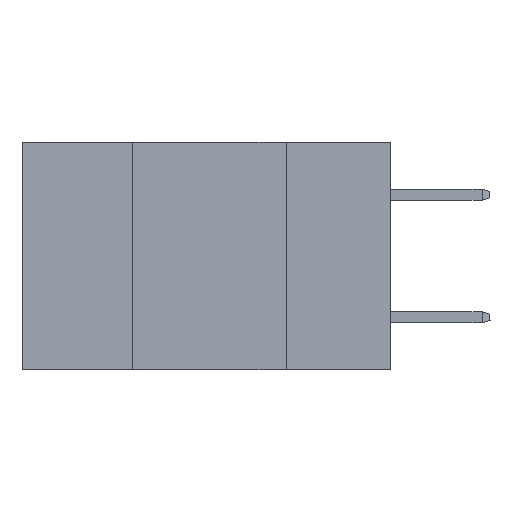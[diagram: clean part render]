
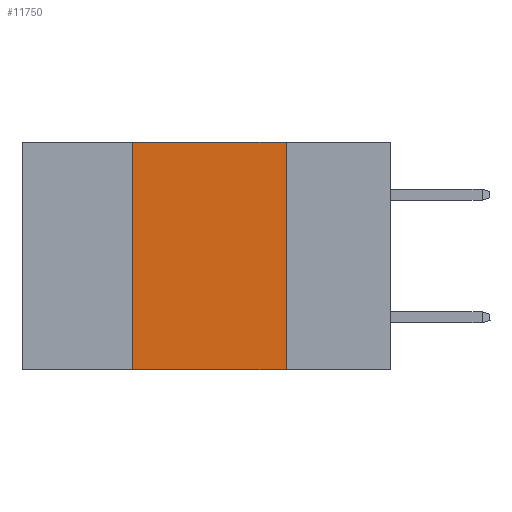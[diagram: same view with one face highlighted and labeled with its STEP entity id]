
A CAD part, left-side view. The second image highlights one B-rep face of the part: STEP entity #11750.
In plain terms, the highlighted planar face has unit normal (-1, 0, 0).
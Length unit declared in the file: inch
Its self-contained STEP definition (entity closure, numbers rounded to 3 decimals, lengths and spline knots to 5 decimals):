
#91 = VERTEX_POINT ( 'NONE', #8208 ) ;
#491 = VECTOR ( 'NONE', #9722, 39.37008 ) ;
#509 = DIRECTION ( 'NONE',  ( 0., -1., 0. ) ) ;
#1171 = LINE ( 'NONE', #6348, #491 ) ;
#2703 = CARTESIAN_POINT ( 'NONE',  ( 0., 0.6, 0. ) ) ;
#2993 = VECTOR ( 'NONE', #509, 39.37008 ) ;
#3059 = DIRECTION ( 'NONE',  ( 0., 0., 1. ) ) ;
#3501 = AXIS2_PLACEMENT_3D ( 'NONE', #6373, #5384, #10749 ) ;
#3661 = VERTEX_POINT ( 'NONE', #12214 ) ;
#5212 = VERTEX_POINT ( 'NONE', #7196 ) ;
#5314 = EDGE_CURVE ( 'NONE', #91, #3661, #13620, .T. ) ;
#5384 = DIRECTION ( 'NONE',  ( 1., 0., 0. ) ) ;
#5668 = PLANE ( 'NONE',  #3501 ) ;
#6065 = EDGE_CURVE ( 'NONE', #3661, #7696, #1171, .T. ) ;
#6348 = CARTESIAN_POINT ( 'NONE',  ( 0., 0.17, 0. ) ) ;
#6373 = CARTESIAN_POINT ( 'NONE',  ( 0., 0.6, 0. ) ) ;
#6686 = ORIENTED_EDGE ( 'NONE', *, *, #10140, .T. ) ;
#7186 = CARTESIAN_POINT ( 'NONE',  ( 0., 0.17, -0.37 ) ) ;
#7196 = CARTESIAN_POINT ( 'NONE',  ( 0., 0.42, -0.37 ) ) ;
#7440 = LINE ( 'NONE', #13830, #12076 ) ;
#7696 = VERTEX_POINT ( 'NONE', #7186 ) ;
#7822 = ORIENTED_EDGE ( 'NONE', *, *, #8713, .F. ) ;
#7993 = VECTOR ( 'NONE', #13829, 39.37008 ) ;
#8208 = CARTESIAN_POINT ( 'NONE',  ( 0., 0.42, 0. ) ) ;
#8713 = EDGE_CURVE ( 'NONE', #5212, #91, #7440, .T. ) ;
#9385 = CARTESIAN_POINT ( 'NONE',  ( 0., 0.6, -0.37 ) ) ;
#9722 = DIRECTION ( 'NONE',  ( 0., 0., -1. ) ) ;
#10140 = EDGE_CURVE ( 'NONE', #5212, #7696, #11594, .T. ) ;
#10749 = DIRECTION ( 'NONE',  ( 0., 0., -1. ) ) ;
#11594 = LINE ( 'NONE', #9385, #7993 ) ;
#11750 = ADVANCED_FACE ( 'NONE', ( #11816 ), #5668, .F. ) ;
#11816 = FACE_OUTER_BOUND ( 'NONE', #13566, .T. ) ;
#12076 = VECTOR ( 'NONE', #3059, 39.37008 ) ;
#12214 = CARTESIAN_POINT ( 'NONE',  ( 0., 0.17, 0. ) ) ;
#12694 = ORIENTED_EDGE ( 'NONE', *, *, #5314, .F. ) ;
#13316 = ORIENTED_EDGE ( 'NONE', *, *, #6065, .F. ) ;
#13566 = EDGE_LOOP ( 'NONE', ( #13316, #12694, #7822, #6686 ) ) ;
#13620 = LINE ( 'NONE', #2703, #2993 ) ;
#13829 = DIRECTION ( 'NONE',  ( 0., -1., 0. ) ) ;
#13830 = CARTESIAN_POINT ( 'NONE',  ( 0., 0.42, 0. ) ) ;
